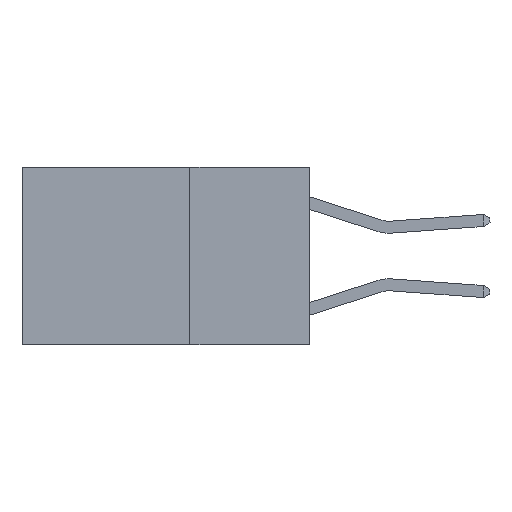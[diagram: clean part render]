
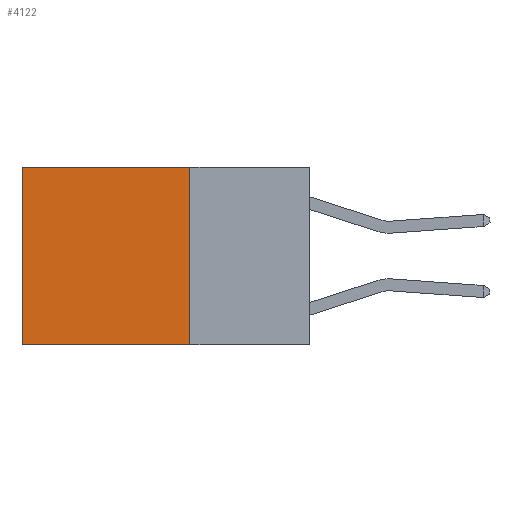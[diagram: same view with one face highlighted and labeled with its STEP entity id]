
A CAD part, left-side view. The second image highlights one B-rep face of the part: STEP entity #4122.
In plain terms, the highlighted planar face has unit normal (-1, 0, 0).
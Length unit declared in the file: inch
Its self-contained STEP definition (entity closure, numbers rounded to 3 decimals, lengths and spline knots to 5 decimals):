
#626 = CARTESIAN_POINT ( 'NONE',  ( 0.2625, 0.25, 0. ) ) ;
#743 = EDGE_LOOP ( 'NONE', ( #10069, #10973, #9185, #12417 ) ) ;
#774 = CARTESIAN_POINT ( 'NONE',  ( 0.2625, 0.6, 0. ) ) ;
#2314 = FACE_OUTER_BOUND ( 'NONE', #743, .T. ) ;
#2749 = LINE ( 'NONE', #12457, #5399 ) ;
#2869 = VERTEX_POINT ( 'NONE', #3265 ) ;
#2905 = LINE ( 'NONE', #3227, #13208 ) ;
#2975 = LINE ( 'NONE', #5384, #6704 ) ;
#3227 = CARTESIAN_POINT ( 'NONE',  ( 0.2625, 0.25, 0. ) ) ;
#3265 = CARTESIAN_POINT ( 'NONE',  ( 0.2625, 0.6, 0. ) ) ;
#4122 = ADVANCED_FACE ( 'NONE', ( #2314 ), #4807, .F. ) ;
#4409 = DIRECTION ( 'NONE',  ( 0., 1., 0. ) ) ;
#4488 = VERTEX_POINT ( 'NONE', #626 ) ;
#4807 = PLANE ( 'NONE',  #12098 ) ;
#5268 = EDGE_CURVE ( 'NONE', #2869, #9324, #12045, .T. ) ;
#5384 = CARTESIAN_POINT ( 'NONE',  ( 0.2625, 0.25, -0.37 ) ) ;
#5399 = VECTOR ( 'NONE', #14683, 39.37008 ) ;
#6015 = EDGE_CURVE ( 'NONE', #10400, #9324, #2975, .T. ) ;
#6050 = CARTESIAN_POINT ( 'NONE',  ( 0.2625, 0.25, 0. ) ) ;
#6704 = VECTOR ( 'NONE', #13348, 39.37008 ) ;
#6852 = CARTESIAN_POINT ( 'NONE',  ( 0.2625, 0.25, -0.37 ) ) ;
#7796 = EDGE_CURVE ( 'NONE', #4488, #10400, #2749, .T. ) ;
#8555 = EDGE_CURVE ( 'NONE', #4488, #2869, #2905, .T. ) ;
#9185 = ORIENTED_EDGE ( 'NONE', *, *, #7796, .F. ) ;
#9324 = VERTEX_POINT ( 'NONE', #14667 ) ;
#10069 = ORIENTED_EDGE ( 'NONE', *, *, #5268, .T. ) ;
#10400 = VERTEX_POINT ( 'NONE', #6852 ) ;
#10501 = DIRECTION ( 'NONE',  ( 0., 0., -1. ) ) ;
#10973 = ORIENTED_EDGE ( 'NONE', *, *, #6015, .F. ) ;
#11586 = DIRECTION ( 'NONE',  ( 1., 0., 0. ) ) ;
#12045 = LINE ( 'NONE', #774, #13628 ) ;
#12098 = AXIS2_PLACEMENT_3D ( 'NONE', #6050, #11586, #10501 ) ;
#12417 = ORIENTED_EDGE ( 'NONE', *, *, #8555, .T. ) ;
#12457 = CARTESIAN_POINT ( 'NONE',  ( 0.2625, 0.25, 0. ) ) ;
#13208 = VECTOR ( 'NONE', #4409, 39.37008 ) ;
#13348 = DIRECTION ( 'NONE',  ( 0., 1., 0. ) ) ;
#13628 = VECTOR ( 'NONE', #14284, 39.37008 ) ;
#14284 = DIRECTION ( 'NONE',  ( 0., 0., -1. ) ) ;
#14667 = CARTESIAN_POINT ( 'NONE',  ( 0.2625, 0.6, -0.37 ) ) ;
#14683 = DIRECTION ( 'NONE',  ( 0., 0., -1. ) ) ;
